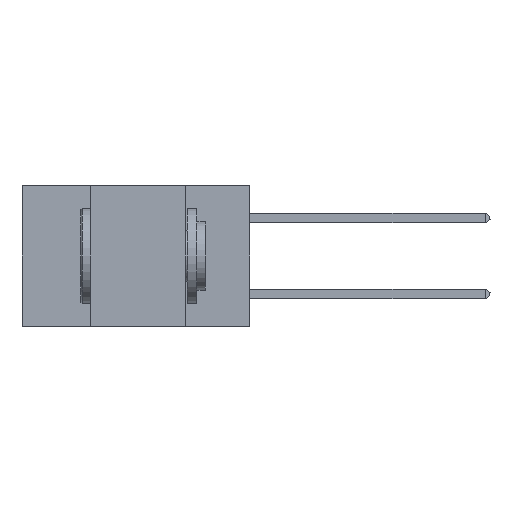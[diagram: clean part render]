
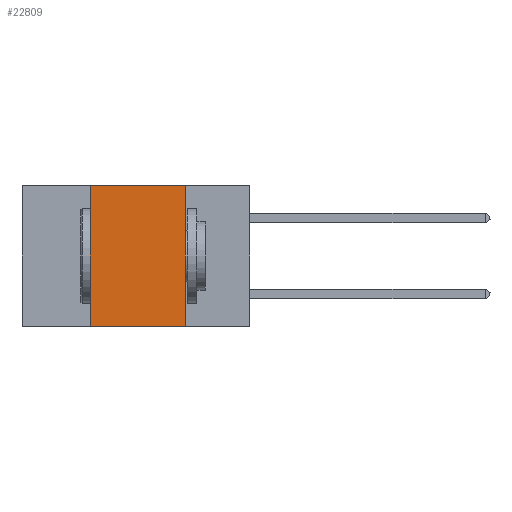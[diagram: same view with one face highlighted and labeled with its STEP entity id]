
A CAD part, left-side view. The second image highlights one B-rep face of the part: STEP entity #22809.
In plain terms, the highlighted planar face has unit normal (-1, 0, 0).
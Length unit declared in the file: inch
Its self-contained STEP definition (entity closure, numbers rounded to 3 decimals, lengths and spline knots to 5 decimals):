
#71 = VECTOR ( 'NONE', #21115, 39.37008 ) ;
#544 = DIRECTION ( 'NONE',  ( 0., 0., -1. ) ) ;
#1406 = DIRECTION ( 'NONE',  ( 0., -1., 0. ) ) ;
#1523 = DIRECTION ( 'NONE',  ( 0., -1., 0. ) ) ;
#2500 = LINE ( 'NONE', #7020, #18843 ) ;
#4157 = ORIENTED_EDGE ( 'NONE', *, *, #16703, .F. ) ;
#4781 = EDGE_CURVE ( 'NONE', #8303, #11352, #2500, .T. ) ;
#7020 = CARTESIAN_POINT ( 'NONE',  ( 0., 0.42, 0. ) ) ;
#7249 = VECTOR ( 'NONE', #1406, 39.37008 ) ;
#7464 = FACE_OUTER_BOUND ( 'NONE', #15398, .T. ) ;
#8303 = VERTEX_POINT ( 'NONE', #10794 ) ;
#8378 = VECTOR ( 'NONE', #1523, 39.37008 ) ;
#9297 = ORIENTED_EDGE ( 'NONE', *, *, #14786, .F. ) ;
#9536 = DIRECTION ( 'NONE',  ( 1., 0., 0. ) ) ;
#9886 = CARTESIAN_POINT ( 'NONE',  ( 0., 0.17, -0.37 ) ) ;
#10272 = CARTESIAN_POINT ( 'NONE',  ( 0., 0.42, 0. ) ) ;
#10485 = CARTESIAN_POINT ( 'NONE',  ( 0., 0.17, 0. ) ) ;
#10794 = CARTESIAN_POINT ( 'NONE',  ( 0., 0.42, -0.37 ) ) ;
#11352 = VERTEX_POINT ( 'NONE', #10272 ) ;
#12073 = DIRECTION ( 'NONE',  ( 0., 0., 1. ) ) ;
#13149 = LINE ( 'NONE', #21117, #7249 ) ;
#14197 = VERTEX_POINT ( 'NONE', #9886 ) ;
#14370 = EDGE_CURVE ( 'NONE', #8303, #14197, #16273, .T. ) ;
#14586 = ORIENTED_EDGE ( 'NONE', *, *, #4781, .F. ) ;
#14786 = EDGE_CURVE ( 'NONE', #11352, #16138, #13149, .T. ) ;
#15307 = LINE ( 'NONE', #21202, #71 ) ;
#15398 = EDGE_LOOP ( 'NONE', ( #4157, #9297, #14586, #20714 ) ) ;
#16138 = VERTEX_POINT ( 'NONE', #10485 ) ;
#16273 = LINE ( 'NONE', #19637, #8378 ) ;
#16494 = CARTESIAN_POINT ( 'NONE',  ( 0., 0.6, 0. ) ) ;
#16703 = EDGE_CURVE ( 'NONE', #16138, #14197, #15307, .T. ) ;
#16731 = PLANE ( 'NONE',  #21785 ) ;
#18843 = VECTOR ( 'NONE', #12073, 39.37008 ) ;
#19637 = CARTESIAN_POINT ( 'NONE',  ( 0., 0.6, -0.37 ) ) ;
#20714 = ORIENTED_EDGE ( 'NONE', *, *, #14370, .T. ) ;
#21115 = DIRECTION ( 'NONE',  ( 0., 0., -1. ) ) ;
#21117 = CARTESIAN_POINT ( 'NONE',  ( 0., 0.6, 0. ) ) ;
#21202 = CARTESIAN_POINT ( 'NONE',  ( 0., 0.17, 0. ) ) ;
#21785 = AXIS2_PLACEMENT_3D ( 'NONE', #16494, #9536, #544 ) ;
#22809 = ADVANCED_FACE ( 'NONE', ( #7464 ), #16731, .F. ) ;
